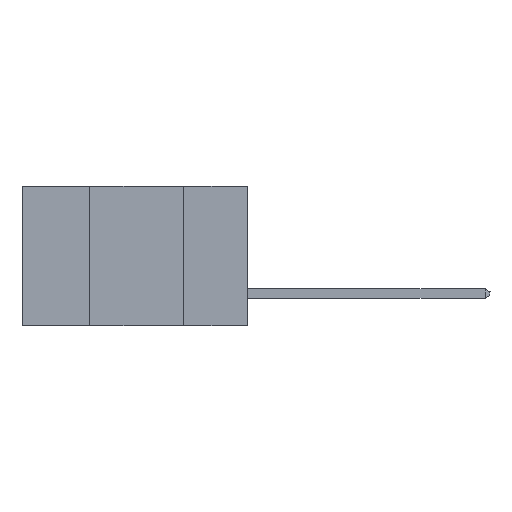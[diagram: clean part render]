
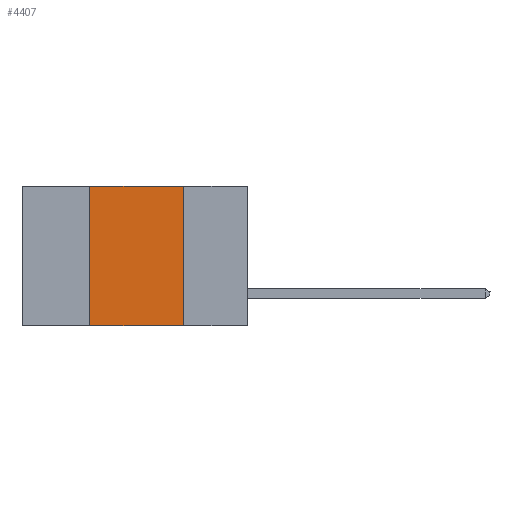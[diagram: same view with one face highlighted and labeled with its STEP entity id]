
A CAD part, left-side view. The second image highlights one B-rep face of the part: STEP entity #4407.
In plain terms, the highlighted planar face has unit normal (-1, 0, 0).
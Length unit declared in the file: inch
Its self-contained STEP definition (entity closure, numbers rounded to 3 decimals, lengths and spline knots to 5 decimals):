
#197 = VECTOR ( 'NONE', #9077, 39.37008 ) ;
#233 = VERTEX_POINT ( 'NONE', #10709 ) ;
#239 = CARTESIAN_POINT ( 'NONE',  ( 0., 0.6, 0. ) ) ;
#262 = DIRECTION ( 'NONE',  ( 0., 0., -1. ) ) ;
#331 = DIRECTION ( 'NONE',  ( 1., 0., 0. ) ) ;
#397 = LINE ( 'NONE', #2943, #7931 ) ;
#495 = ORIENTED_EDGE ( 'NONE', *, *, #13673, .F. ) ;
#947 = CARTESIAN_POINT ( 'NONE',  ( 0., 0.17, -0.37 ) ) ;
#1178 = LINE ( 'NONE', #6896, #14146 ) ;
#1581 = CARTESIAN_POINT ( 'NONE',  ( 0., 0.42, -0.37 ) ) ;
#2624 = ORIENTED_EDGE ( 'NONE', *, *, #4046, .F. ) ;
#2943 = CARTESIAN_POINT ( 'NONE',  ( 0., 0.42, -0.37 ) ) ;
#3002 = EDGE_LOOP ( 'NONE', ( #2624, #495, #12242, #7920 ) ) ;
#3236 = EDGE_CURVE ( 'NONE', #14203, #233, #397, .T. ) ;
#3435 = VECTOR ( 'NONE', #10811, 39.37008 ) ;
#3648 = LINE ( 'NONE', #239, #197 ) ;
#4046 = EDGE_CURVE ( 'NONE', #6478, #5478, #1178, .T. ) ;
#4407 = ADVANCED_FACE ( 'NONE', ( #10048 ), #11249, .F. ) ;
#5478 = VERTEX_POINT ( 'NONE', #947 ) ;
#6478 = VERTEX_POINT ( 'NONE', #7825 ) ;
#6896 = CARTESIAN_POINT ( 'NONE',  ( 0., 0.17, -0.37 ) ) ;
#7825 = CARTESIAN_POINT ( 'NONE',  ( 0., 0.17, 0. ) ) ;
#7920 = ORIENTED_EDGE ( 'NONE', *, *, #13408, .T. ) ;
#7931 = VECTOR ( 'NONE', #11673, 39.37008 ) ;
#9077 = DIRECTION ( 'NONE',  ( 0., -1., 0. ) ) ;
#10048 = FACE_OUTER_BOUND ( 'NONE', #3002, .T. ) ;
#10179 = CARTESIAN_POINT ( 'NONE',  ( 0., 0.6, 0. ) ) ;
#10709 = CARTESIAN_POINT ( 'NONE',  ( 0., 0.42, 0. ) ) ;
#10811 = DIRECTION ( 'NONE',  ( 0., -1., 0. ) ) ;
#11249 = PLANE ( 'NONE',  #13460 ) ;
#11280 = DIRECTION ( 'NONE',  ( 0., 0., -1. ) ) ;
#11673 = DIRECTION ( 'NONE',  ( 0., 0., 1. ) ) ;
#11815 = CARTESIAN_POINT ( 'NONE',  ( 0., 0.6, -0.37 ) ) ;
#12242 = ORIENTED_EDGE ( 'NONE', *, *, #3236, .F. ) ;
#12812 = LINE ( 'NONE', #11815, #3435 ) ;
#13408 = EDGE_CURVE ( 'NONE', #14203, #5478, #12812, .T. ) ;
#13460 = AXIS2_PLACEMENT_3D ( 'NONE', #10179, #331, #262 ) ;
#13673 = EDGE_CURVE ( 'NONE', #233, #6478, #3648, .T. ) ;
#14146 = VECTOR ( 'NONE', #11280, 39.37008 ) ;
#14203 = VERTEX_POINT ( 'NONE', #1581 ) ;
